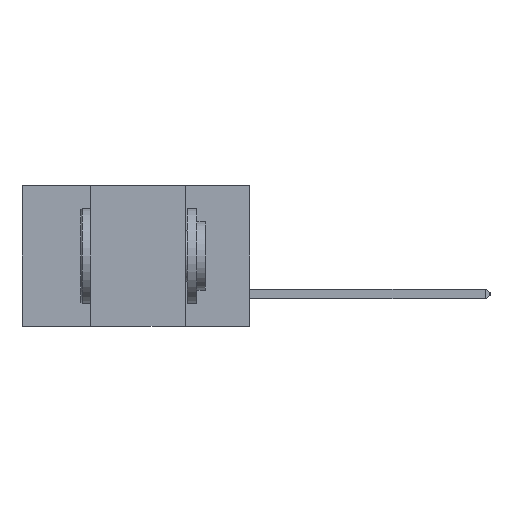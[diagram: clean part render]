
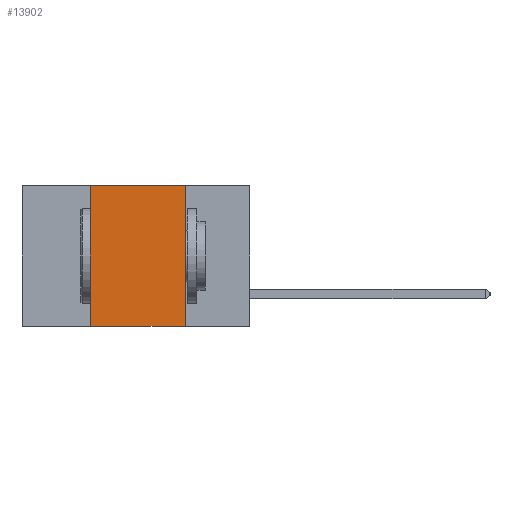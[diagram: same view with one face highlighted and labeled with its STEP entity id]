
A CAD part, left-side view. The second image highlights one B-rep face of the part: STEP entity #13902.
In plain terms, the highlighted planar face has unit normal (-1, 0, 0).
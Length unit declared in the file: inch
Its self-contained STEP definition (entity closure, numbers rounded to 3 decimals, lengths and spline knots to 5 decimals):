
#359 = CARTESIAN_POINT ( 'NONE',  ( 0., 0.17, -0.37 ) ) ;
#374 = CARTESIAN_POINT ( 'NONE',  ( 0., 0.42, -0.37 ) ) ;
#666 = VECTOR ( 'NONE', #7209, 39.37008 ) ;
#1086 = LINE ( 'NONE', #13940, #666 ) ;
#1438 = PLANE ( 'NONE',  #2541 ) ;
#2016 = VERTEX_POINT ( 'NONE', #359 ) ;
#2541 = AXIS2_PLACEMENT_3D ( 'NONE', #10958, #12314, #4207 ) ;
#2806 = VERTEX_POINT ( 'NONE', #7291 ) ;
#3285 = LINE ( 'NONE', #5396, #10488 ) ;
#3940 = FACE_OUTER_BOUND ( 'NONE', #17009, .T. ) ;
#3945 = ORIENTED_EDGE ( 'NONE', *, *, #7667, .F. ) ;
#4049 = LINE ( 'NONE', #12452, #14430 ) ;
#4207 = DIRECTION ( 'NONE',  ( 0., 0., -1. ) ) ;
#4537 = VERTEX_POINT ( 'NONE', #374 ) ;
#5396 = CARTESIAN_POINT ( 'NONE',  ( 0., 0.6, -0.37 ) ) ;
#5952 = ORIENTED_EDGE ( 'NONE', *, *, #6566, .F. ) ;
#5989 = EDGE_CURVE ( 'NONE', #2806, #8873, #7075, .T. ) ;
#6566 = EDGE_CURVE ( 'NONE', #4537, #2806, #1086, .T. ) ;
#6642 = VECTOR ( 'NONE', #11300, 39.37008 ) ;
#7075 = LINE ( 'NONE', #9923, #6642 ) ;
#7209 = DIRECTION ( 'NONE',  ( 0., 0., 1. ) ) ;
#7291 = CARTESIAN_POINT ( 'NONE',  ( 0., 0.42, 0. ) ) ;
#7649 = ORIENTED_EDGE ( 'NONE', *, *, #5989, .F. ) ;
#7667 = EDGE_CURVE ( 'NONE', #8873, #2016, #4049, .T. ) ;
#8132 = EDGE_CURVE ( 'NONE', #4537, #2016, #3285, .T. ) ;
#8873 = VERTEX_POINT ( 'NONE', #12781 ) ;
#9923 = CARTESIAN_POINT ( 'NONE',  ( 0., 0.6, 0. ) ) ;
#10488 = VECTOR ( 'NONE', #14863, 39.37008 ) ;
#10958 = CARTESIAN_POINT ( 'NONE',  ( 0., 0.6, 0. ) ) ;
#11239 = ORIENTED_EDGE ( 'NONE', *, *, #8132, .T. ) ;
#11300 = DIRECTION ( 'NONE',  ( 0., -1., 0. ) ) ;
#12314 = DIRECTION ( 'NONE',  ( 1., 0., 0. ) ) ;
#12452 = CARTESIAN_POINT ( 'NONE',  ( 0., 0.17, 0. ) ) ;
#12781 = CARTESIAN_POINT ( 'NONE',  ( 0., 0.17, 0. ) ) ;
#13902 = ADVANCED_FACE ( 'NONE', ( #3940 ), #1438, .F. ) ;
#13940 = CARTESIAN_POINT ( 'NONE',  ( 0., 0.42, 0. ) ) ;
#14430 = VECTOR ( 'NONE', #15127, 39.37008 ) ;
#14863 = DIRECTION ( 'NONE',  ( 0., -1., 0. ) ) ;
#15127 = DIRECTION ( 'NONE',  ( 0., 0., -1. ) ) ;
#17009 = EDGE_LOOP ( 'NONE', ( #3945, #7649, #5952, #11239 ) ) ;
